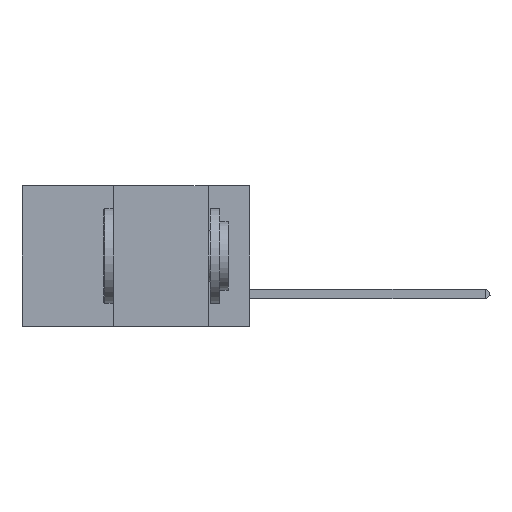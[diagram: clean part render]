
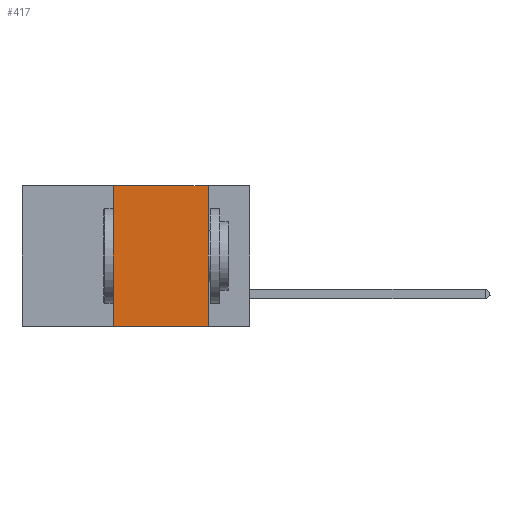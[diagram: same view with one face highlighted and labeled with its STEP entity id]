
A CAD part, left-side view. The second image highlights one B-rep face of the part: STEP entity #417.
In plain terms, the highlighted planar face has unit normal (-1, 0, 0).
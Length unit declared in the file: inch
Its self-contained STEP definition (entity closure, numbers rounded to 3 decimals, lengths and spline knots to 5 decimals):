
#417 = ADVANCED_FACE ( 'NONE', ( #12177 ), #14748, .F. ) ;
#635 = LINE ( 'NONE', #7656, #15708 ) ;
#1338 = DIRECTION ( 'NONE',  ( 0., 0., -1. ) ) ;
#1659 = VERTEX_POINT ( 'NONE', #3625 ) ;
#1963 = VERTEX_POINT ( 'NONE', #18014 ) ;
#2167 = ORIENTED_EDGE ( 'NONE', *, *, #14265, .T. ) ;
#3625 = CARTESIAN_POINT ( 'NONE',  ( 0., 0.11, -0.37 ) ) ;
#4894 = DIRECTION ( 'NONE',  ( 0., 0., -1. ) ) ;
#5728 = VECTOR ( 'NONE', #1338, 39.37008 ) ;
#5757 = CARTESIAN_POINT ( 'NONE',  ( 0., 0.36, -0.37 ) ) ;
#7656 = CARTESIAN_POINT ( 'NONE',  ( 0., 0.6, -0.37 ) ) ;
#7819 = VERTEX_POINT ( 'NONE', #5757 ) ;
#8713 = CARTESIAN_POINT ( 'NONE',  ( 0., 0.11, 0. ) ) ;
#9665 = DIRECTION ( 'NONE',  ( 0., 0., 1. ) ) ;
#9841 = DIRECTION ( 'NONE',  ( 1., 0., 0. ) ) ;
#9872 = ORIENTED_EDGE ( 'NONE', *, *, #14426, .F. ) ;
#11228 = DIRECTION ( 'NONE',  ( 0., -1., 0. ) ) ;
#11987 = LINE ( 'NONE', #13071, #19693 ) ;
#12177 = FACE_OUTER_BOUND ( 'NONE', #19484, .T. ) ;
#13034 = LINE ( 'NONE', #14806, #14389 ) ;
#13071 = CARTESIAN_POINT ( 'NONE',  ( 0., 0.36, 0. ) ) ;
#13105 = CARTESIAN_POINT ( 'NONE',  ( 0., 0.6, 0. ) ) ;
#14265 = EDGE_CURVE ( 'NONE', #7819, #1659, #635, .T. ) ;
#14389 = VECTOR ( 'NONE', #20118, 39.37008 ) ;
#14426 = EDGE_CURVE ( 'NONE', #1963, #18650, #13034, .T. ) ;
#14748 = PLANE ( 'NONE',  #18090 ) ;
#14806 = CARTESIAN_POINT ( 'NONE',  ( 0., 0.6, 0. ) ) ;
#14941 = CARTESIAN_POINT ( 'NONE',  ( 0., 0.11, 0. ) ) ;
#15708 = VECTOR ( 'NONE', #11228, 39.37008 ) ;
#16827 = LINE ( 'NONE', #14941, #5728 ) ;
#18014 = CARTESIAN_POINT ( 'NONE',  ( 0., 0.36, 0. ) ) ;
#18090 = AXIS2_PLACEMENT_3D ( 'NONE', #13105, #9841, #4894 ) ;
#18302 = ORIENTED_EDGE ( 'NONE', *, *, #19729, .F. ) ;
#18398 = ORIENTED_EDGE ( 'NONE', *, *, #18571, .F. ) ;
#18571 = EDGE_CURVE ( 'NONE', #18650, #1659, #16827, .T. ) ;
#18650 = VERTEX_POINT ( 'NONE', #8713 ) ;
#19484 = EDGE_LOOP ( 'NONE', ( #18398, #9872, #18302, #2167 ) ) ;
#19693 = VECTOR ( 'NONE', #9665, 39.37008 ) ;
#19729 = EDGE_CURVE ( 'NONE', #7819, #1963, #11987, .T. ) ;
#20118 = DIRECTION ( 'NONE',  ( 0., -1., 0. ) ) ;
